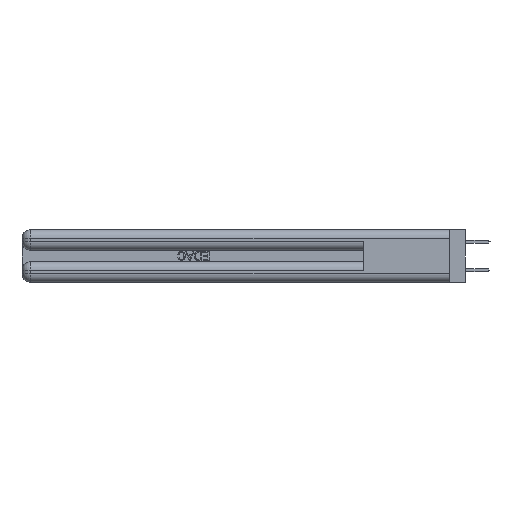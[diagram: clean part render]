
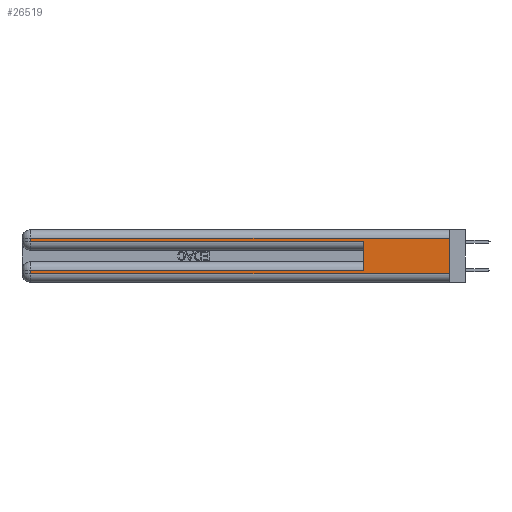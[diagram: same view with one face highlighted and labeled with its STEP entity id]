
A CAD part, left-side view. The second image highlights one B-rep face of the part: STEP entity #26519.
In plain terms, the highlighted planar face has unit normal (-1, 0, 0).
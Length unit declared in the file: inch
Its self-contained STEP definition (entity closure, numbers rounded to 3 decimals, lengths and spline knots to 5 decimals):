
#384 = FACE_OUTER_BOUND ( 'NONE', #22652, .T. ) ;
#792 = VECTOR ( 'NONE', #40726, 39.37008 ) ;
#796 = LINE ( 'NONE', #17125, #25831 ) ;
#1002 = CARTESIAN_POINT ( 'NONE',  ( 0., 0.6, 0.145 ) ) ;
#1167 = VECTOR ( 'NONE', #16925, 39.37008 ) ;
#1298 = DIRECTION ( 'NONE',  ( 0., 0., 1. ) ) ;
#1346 = CARTESIAN_POINT ( 'NONE',  ( 0., 0., 0.085 ) ) ;
#1825 = VECTOR ( 'NONE', #26855, 39.37008 ) ;
#2886 = LINE ( 'NONE', #34665, #26915 ) ;
#3605 = VECTOR ( 'NONE', #11136, 39.37008 ) ;
#5524 = CARTESIAN_POINT ( 'NONE',  ( 0., 2.94, 0.06 ) ) ;
#6027 = VERTEX_POINT ( 'NONE', #16329 ) ;
#6339 = LINE ( 'NONE', #13409, #1825 ) ;
#6812 = DIRECTION ( 'NONE',  ( 0., 0., -1. ) ) ;
#6976 = ORIENTED_EDGE ( 'NONE', *, *, #33968, .T. ) ;
#8607 = DIRECTION ( 'NONE',  ( 0., 0., -1. ) ) ;
#8907 = LINE ( 'NONE', #11659, #792 ) ;
#9770 = LINE ( 'NONE', #29945, #1167 ) ;
#9858 = DIRECTION ( 'NONE',  ( 1., 0., 0. ) ) ;
#11136 = DIRECTION ( 'NONE',  ( 0., 1., 0. ) ) ;
#11659 = CARTESIAN_POINT ( 'NONE',  ( 0., 0., 0.285 ) ) ;
#12198 = DIRECTION ( 'NONE',  ( 0., 0., -1. ) ) ;
#12549 = ORIENTED_EDGE ( 'NONE', *, *, #23158, .T. ) ;
#12850 = CARTESIAN_POINT ( 'NONE',  ( 0., 2.94, 0.085 ) ) ;
#13409 = CARTESIAN_POINT ( 'NONE',  ( 0., 0., 0.06 ) ) ;
#15322 = AXIS2_PLACEMENT_3D ( 'NONE', #20059, #9858, #19910 ) ;
#16329 = CARTESIAN_POINT ( 'NONE',  ( 0., 2.94, 0.31 ) ) ;
#16405 = CARTESIAN_POINT ( 'NONE',  ( 0., 0.6, 0.285 ) ) ;
#16925 = DIRECTION ( 'NONE',  ( 0., 1., 0. ) ) ;
#17125 = CARTESIAN_POINT ( 'NONE',  ( 0., 2.94, 0.37 ) ) ;
#17327 = EDGE_CURVE ( 'NONE', #17718, #31852, #2886, .T. ) ;
#17644 = VERTEX_POINT ( 'NONE', #12850 ) ;
#17718 = VERTEX_POINT ( 'NONE', #25875 ) ;
#18109 = EDGE_CURVE ( 'NONE', #26836, #40078, #8907, .T. ) ;
#19910 = DIRECTION ( 'NONE',  ( 0., 0., -1. ) ) ;
#20059 = CARTESIAN_POINT ( 'NONE',  ( 0., 0., 0.37 ) ) ;
#22573 = VECTOR ( 'NONE', #8607, 39.37008 ) ;
#22652 = EDGE_LOOP ( 'NONE', ( #22859, #40790, #38389, #41587, #26281, #6976, #12549, #26291 ) ) ;
#22859 = ORIENTED_EDGE ( 'NONE', *, *, #17327, .F. ) ;
#23158 = EDGE_CURVE ( 'NONE', #17644, #41457, #24619, .T. ) ;
#23480 = PLANE ( 'NONE',  #15322 ) ;
#24619 = LINE ( 'NONE', #24957, #22573 ) ;
#24957 = CARTESIAN_POINT ( 'NONE',  ( 0., 2.94, 0.37 ) ) ;
#25831 = VECTOR ( 'NONE', #6812, 39.37008 ) ;
#25875 = CARTESIAN_POINT ( 'NONE',  ( 0., 0., 0.31 ) ) ;
#26281 = ORIENTED_EDGE ( 'NONE', *, *, #37660, .F. ) ;
#26291 = ORIENTED_EDGE ( 'NONE', *, *, #37458, .T. ) ;
#26519 = ADVANCED_FACE ( 'NONE', ( #384 ), #23480, .F. ) ;
#26836 = VERTEX_POINT ( 'NONE', #37910 ) ;
#26855 = DIRECTION ( 'NONE',  ( 0., -1., 0. ) ) ;
#26915 = VECTOR ( 'NONE', #12198, 39.37008 ) ;
#27338 = VECTOR ( 'NONE', #1298, 39.37008 ) ;
#27657 = LINE ( 'NONE', #1346, #3605 ) ;
#28987 = EDGE_CURVE ( 'NONE', #17718, #6027, #9770, .T. ) ;
#29100 = CARTESIAN_POINT ( 'NONE',  ( 0., 0.6, 0.085 ) ) ;
#29945 = CARTESIAN_POINT ( 'NONE',  ( 0., 0., 0.31 ) ) ;
#29985 = VERTEX_POINT ( 'NONE', #29100 ) ;
#31852 = VERTEX_POINT ( 'NONE', #35285 ) ;
#33968 = EDGE_CURVE ( 'NONE', #29985, #17644, #27657, .T. ) ;
#34665 = CARTESIAN_POINT ( 'NONE',  ( 0., 0., 0.37 ) ) ;
#35285 = CARTESIAN_POINT ( 'NONE',  ( 0., 0., 0.06 ) ) ;
#36553 = LINE ( 'NONE', #1002, #27338 ) ;
#37458 = EDGE_CURVE ( 'NONE', #41457, #31852, #6339, .T. ) ;
#37472 = EDGE_CURVE ( 'NONE', #6027, #26836, #796, .T. ) ;
#37660 = EDGE_CURVE ( 'NONE', #29985, #40078, #36553, .T. ) ;
#37910 = CARTESIAN_POINT ( 'NONE',  ( 0., 2.94, 0.285 ) ) ;
#38389 = ORIENTED_EDGE ( 'NONE', *, *, #37472, .T. ) ;
#40078 = VERTEX_POINT ( 'NONE', #16405 ) ;
#40726 = DIRECTION ( 'NONE',  ( 0., -1., 0. ) ) ;
#40790 = ORIENTED_EDGE ( 'NONE', *, *, #28987, .T. ) ;
#41457 = VERTEX_POINT ( 'NONE', #5524 ) ;
#41587 = ORIENTED_EDGE ( 'NONE', *, *, #18109, .T. ) ;
